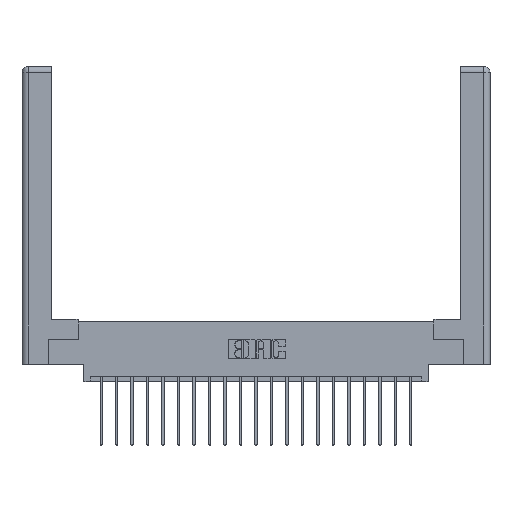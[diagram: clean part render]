
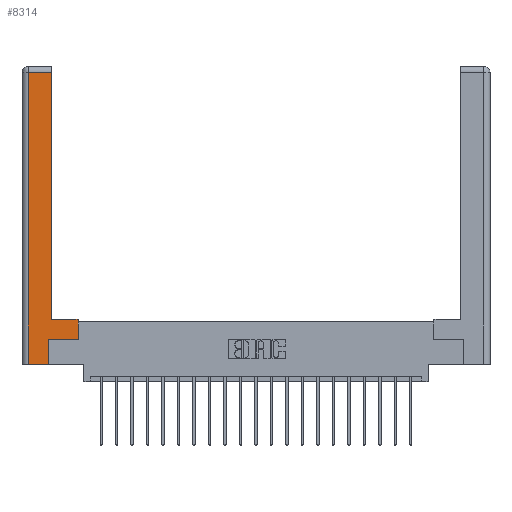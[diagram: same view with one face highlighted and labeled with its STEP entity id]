
A CAD part, top view. The second image highlights one B-rep face of the part: STEP entity #8314.
In plain terms, the highlighted planar face has unit normal (0, 0, 1).
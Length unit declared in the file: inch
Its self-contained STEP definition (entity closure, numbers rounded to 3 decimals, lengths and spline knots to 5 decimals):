
#54 = CARTESIAN_POINT ( 'NONE',  ( 0.295, 0.45, 0. ) ) ;
#240 = VERTEX_POINT ( 'NONE', #11633 ) ;
#490 = CARTESIAN_POINT ( 'NONE',  ( 0.265, 0.245, 0. ) ) ;
#727 = EDGE_CURVE ( 'NONE', #14414, #6013, #6042, .T. ) ;
#952 = CARTESIAN_POINT ( 'NONE',  ( 0.0615, 2.94, 0. ) ) ;
#1182 = VECTOR ( 'NONE', #19341, 39.37008 ) ;
#1384 = DIRECTION ( 'NONE',  ( 1., 0., 0. ) ) ;
#1873 = CARTESIAN_POINT ( 'NONE',  ( 0.265, 0., 0. ) ) ;
#1927 = EDGE_CURVE ( 'NONE', #6958, #9394, #8881, .T. ) ;
#2084 = LINE ( 'NONE', #13737, #17876 ) ;
#2753 = CARTESIAN_POINT ( 'NONE',  ( 0.565, 0.245, 0. ) ) ;
#2844 = CARTESIAN_POINT ( 'NONE',  ( 0.0615, 0., 0. ) ) ;
#3583 = VECTOR ( 'NONE', #10122, 39.37008 ) ;
#4625 = CARTESIAN_POINT ( 'NONE',  ( 0.565, 0.245, 0. ) ) ;
#5054 = AXIS2_PLACEMENT_3D ( 'NONE', #20117, #18461, #6628 ) ;
#5115 = DIRECTION ( 'NONE',  ( -1., 0., 0. ) ) ;
#5770 = EDGE_CURVE ( 'NONE', #6047, #6958, #18451, .T. ) ;
#5860 = LINE ( 'NONE', #13411, #14284 ) ;
#6013 = VERTEX_POINT ( 'NONE', #16371 ) ;
#6042 = LINE ( 'NONE', #6725, #19465 ) ;
#6047 = VERTEX_POINT ( 'NONE', #952 ) ;
#6323 = ORIENTED_EDGE ( 'NONE', *, *, #727, .T. ) ;
#6628 = DIRECTION ( 'NONE',  ( -1., 0., 0. ) ) ;
#6694 = CARTESIAN_POINT ( 'NONE',  ( 0.0615, 0., 0. ) ) ;
#6725 = CARTESIAN_POINT ( 'NONE',  ( 0.295, 3., 0. ) ) ;
#6935 = CARTESIAN_POINT ( 'NONE',  ( 0.265, 0., 0. ) ) ;
#6958 = VERTEX_POINT ( 'NONE', #2844 ) ;
#7677 = ORIENTED_EDGE ( 'NONE', *, *, #20071, .T. ) ;
#8066 = VERTEX_POINT ( 'NONE', #490 ) ;
#8140 = EDGE_LOOP ( 'NONE', ( #6323, #7677, #11450, #9369, #9799, #18683, #8142, #11006 ) ) ;
#8142 = ORIENTED_EDGE ( 'NONE', *, *, #14319, .T. ) ;
#8314 = ADVANCED_FACE ( 'NONE', ( #20570 ), #11722, .F. ) ;
#8339 = DIRECTION ( 'NONE',  ( 0., 1., 0. ) ) ;
#8881 = LINE ( 'NONE', #6935, #10183 ) ;
#9369 = ORIENTED_EDGE ( 'NONE', *, *, #1927, .T. ) ;
#9394 = VERTEX_POINT ( 'NONE', #1873 ) ;
#9799 = ORIENTED_EDGE ( 'NONE', *, *, #12254, .T. ) ;
#10054 = VERTEX_POINT ( 'NONE', #4625 ) ;
#10122 = DIRECTION ( 'NONE',  ( 0., 1., 0. ) ) ;
#10183 = VECTOR ( 'NONE', #1384, 39.37008 ) ;
#11006 = ORIENTED_EDGE ( 'NONE', *, *, #17033, .T. ) ;
#11450 = ORIENTED_EDGE ( 'NONE', *, *, #5770, .T. ) ;
#11633 = CARTESIAN_POINT ( 'NONE',  ( 0.565, 0.45, 0. ) ) ;
#11658 = CARTESIAN_POINT ( 'NONE',  ( 0.265, 0.245, 0. ) ) ;
#11722 = PLANE ( 'NONE',  #5054 ) ;
#12254 = EDGE_CURVE ( 'NONE', #9394, #8066, #20052, .T. ) ;
#13411 = CARTESIAN_POINT ( 'NONE',  ( 0.295, 0.45, 0. ) ) ;
#13476 = DIRECTION ( 'NONE',  ( 0., -1., 0. ) ) ;
#13737 = CARTESIAN_POINT ( 'NONE',  ( 0.0615, 2.94, 0. ) ) ;
#14284 = VECTOR ( 'NONE', #16992, 39.37008 ) ;
#14319 = EDGE_CURVE ( 'NONE', #10054, #240, #18081, .T. ) ;
#14414 = VERTEX_POINT ( 'NONE', #54 ) ;
#14512 = VECTOR ( 'NONE', #8339, 39.37008 ) ;
#15128 = EDGE_CURVE ( 'NONE', #8066, #10054, #19102, .T. ) ;
#16371 = CARTESIAN_POINT ( 'NONE',  ( 0.295, 2.94, 0. ) ) ;
#16992 = DIRECTION ( 'NONE',  ( -1., 0., 0. ) ) ;
#17033 = EDGE_CURVE ( 'NONE', #240, #14414, #5860, .T. ) ;
#17326 = DIRECTION ( 'NONE',  ( 0., 1., 0. ) ) ;
#17876 = VECTOR ( 'NONE', #5115, 39.37008 ) ;
#18081 = LINE ( 'NONE', #18406, #3583 ) ;
#18406 = CARTESIAN_POINT ( 'NONE',  ( 0.565, 0.45, 0. ) ) ;
#18451 = LINE ( 'NONE', #6694, #18710 ) ;
#18461 = DIRECTION ( 'NONE',  ( 0., 0., -1. ) ) ;
#18683 = ORIENTED_EDGE ( 'NONE', *, *, #15128, .T. ) ;
#18710 = VECTOR ( 'NONE', #13476, 39.37008 ) ;
#19102 = LINE ( 'NONE', #2753, #1182 ) ;
#19341 = DIRECTION ( 'NONE',  ( 1., 0., 0. ) ) ;
#19465 = VECTOR ( 'NONE', #17326, 39.37008 ) ;
#20052 = LINE ( 'NONE', #11658, #14512 ) ;
#20071 = EDGE_CURVE ( 'NONE', #6013, #6047, #2084, .T. ) ;
#20117 = CARTESIAN_POINT ( 'NONE',  ( 0., 0., 0. ) ) ;
#20570 = FACE_OUTER_BOUND ( 'NONE', #8140, .T. ) ;
